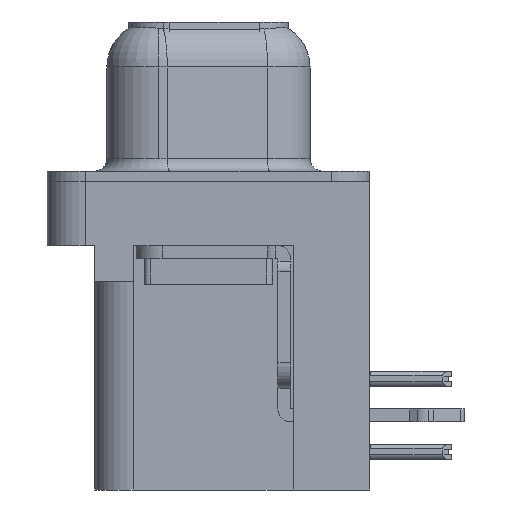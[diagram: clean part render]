
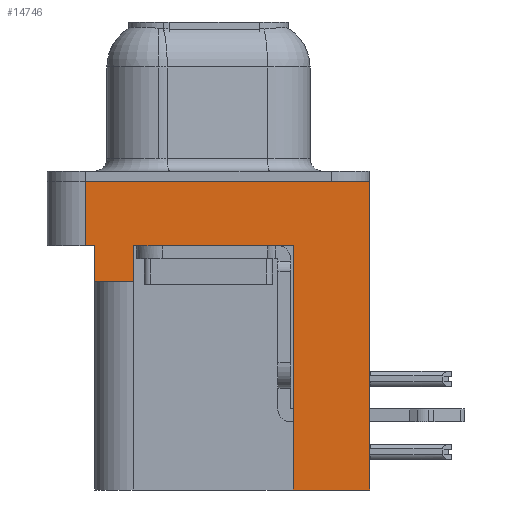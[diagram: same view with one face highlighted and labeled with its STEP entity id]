
A CAD part, left-side view. The second image highlights one B-rep face of the part: STEP entity #14746.
In plain terms, the highlighted planar face has unit normal (-1, 0, 0).
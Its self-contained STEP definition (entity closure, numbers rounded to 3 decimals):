
#140 = CARTESIAN_POINT ( 'NONE',  ( -2.935, -3.295, -2.5 ) ) ;
#238 = DIRECTION ( 'NONE',  ( 0., 0., 1. ) ) ;
#507 = LINE ( 'NONE', #5532, #8918 ) ;
#726 = CARTESIAN_POINT ( 'NONE',  ( -2.935, -6.275, -2.5 ) ) ;
#1962 = VERTEX_POINT ( 'NONE', #24941 ) ;
#2239 = VERTEX_POINT ( 'NONE', #6977 ) ;
#2416 = ORIENTED_EDGE ( 'NONE', *, *, #14369, .F. ) ;
#2509 = EDGE_CURVE ( 'NONE', #13848, #7947, #21451, .T. ) ;
#2587 = LINE ( 'NONE', #9626, #4948 ) ;
#2781 = VECTOR ( 'NONE', #238, 1000. ) ;
#2790 = LINE ( 'NONE', #20715, #17519 ) ;
#3121 = ORIENTED_EDGE ( 'NONE', *, *, #6282, .T. ) ;
#3251 = CARTESIAN_POINT ( 'NONE',  ( -2.935, -3.295, -12. ) ) ;
#3507 = DIRECTION ( 'NONE',  ( 0., 1., 0. ) ) ;
#3618 = VECTOR ( 'NONE', #19946, 1000. ) ;
#3640 = CARTESIAN_POINT ( 'NONE',  ( -2.935, 2.895, -2.5 ) ) ;
#3683 = DIRECTION ( 'NONE',  ( 0., 0., 1. ) ) ;
#3917 = EDGE_CURVE ( 'NONE', #13127, #20764, #21679, .T. ) ;
#4265 = DIRECTION ( 'NONE',  ( 0., 0., 1. ) ) ;
#4433 = PLANE ( 'NONE',  #15944 ) ;
#4751 = LINE ( 'NONE', #10506, #11701 ) ;
#4853 = CARTESIAN_POINT ( 'NONE',  ( -2.935, 4.425, -3.9 ) ) ;
#4948 = VECTOR ( 'NONE', #19466, 1000. ) ;
#5463 = CARTESIAN_POINT ( 'NONE',  ( -2.935, 4.775, -2.5 ) ) ;
#5532 = CARTESIAN_POINT ( 'NONE',  ( -2.935, -6.275, -2.5 ) ) ;
#6073 = EDGE_CURVE ( 'NONE', #7947, #1962, #8695, .T. ) ;
#6282 = EDGE_CURVE ( 'NONE', #13848, #2239, #4751, .T. ) ;
#6315 = ORIENTED_EDGE ( 'NONE', *, *, #17492, .T. ) ;
#6928 = EDGE_LOOP ( 'NONE', ( #19329, #10002, #3121, #24791, #21638, #9398, #6315, #24312, #2416, #16852 ) ) ;
#6977 = CARTESIAN_POINT ( 'NONE',  ( -2.935, 4.425, -2.5 ) ) ;
#7828 = CARTESIAN_POINT ( 'NONE',  ( -2.935, 4.775, -2.5 ) ) ;
#7875 = VECTOR ( 'NONE', #22246, 1000. ) ;
#7947 = VERTEX_POINT ( 'NONE', #19661 ) ;
#8245 = LINE ( 'NONE', #18409, #19979 ) ;
#8695 = LINE ( 'NONE', #10614, #3618 ) ;
#8802 = CARTESIAN_POINT ( 'NONE',  ( -2.935, 4.425, -3.9 ) ) ;
#8918 = VECTOR ( 'NONE', #3683, 1000. ) ;
#9371 = FACE_OUTER_BOUND ( 'NONE', #6928, .T. ) ;
#9398 = ORIENTED_EDGE ( 'NONE', *, *, #3917, .T. ) ;
#9626 = CARTESIAN_POINT ( 'NONE',  ( -2.935, -3.295, -12. ) ) ;
#9820 = DIRECTION ( 'NONE',  ( 0., 0., 1. ) ) ;
#10002 = ORIENTED_EDGE ( 'NONE', *, *, #2509, .F. ) ;
#10506 = CARTESIAN_POINT ( 'NONE',  ( -2.935, -6.275, -2.5 ) ) ;
#10614 = CARTESIAN_POINT ( 'NONE',  ( -2.935, -6.275, 0. ) ) ;
#11242 = VECTOR ( 'NONE', #9820, 1000. ) ;
#11701 = VECTOR ( 'NONE', #18063, 1000. ) ;
#12180 = CARTESIAN_POINT ( 'NONE',  ( -2.935, -6.275, -12. ) ) ;
#13011 = LINE ( 'NONE', #8802, #7875 ) ;
#13127 = VERTEX_POINT ( 'NONE', #13925 ) ;
#13670 = CARTESIAN_POINT ( 'NONE',  ( -2.935, 2.895, -3.9 ) ) ;
#13848 = VERTEX_POINT ( 'NONE', #7828 ) ;
#13925 = CARTESIAN_POINT ( 'NONE',  ( -2.935, 2.895, -3.9 ) ) ;
#14369 = EDGE_CURVE ( 'NONE', #18572, #18640, #2790, .T. ) ;
#14418 = VERTEX_POINT ( 'NONE', #140 ) ;
#14746 = ADVANCED_FACE ( 'NONE', ( #9371 ), #4433, .T. ) ;
#15848 = DIRECTION ( 'NONE',  ( -1., 0., 0. ) ) ;
#15944 = AXIS2_PLACEMENT_3D ( 'NONE', #726, #15848, #4265 ) ;
#16317 = EDGE_CURVE ( 'NONE', #18572, #1962, #507, .T. ) ;
#16359 = EDGE_CURVE ( 'NONE', #18640, #14418, #2587, .T. ) ;
#16845 = DIRECTION ( 'NONE',  ( 0., 1., 0. ) ) ;
#16852 = ORIENTED_EDGE ( 'NONE', *, *, #16317, .T. ) ;
#17492 = EDGE_CURVE ( 'NONE', #20764, #14418, #8245, .T. ) ;
#17519 = VECTOR ( 'NONE', #3507, 1000. ) ;
#18063 = DIRECTION ( 'NONE',  ( 0., -1., 0. ) ) ;
#18361 = VECTOR ( 'NONE', #16845, 1000. ) ;
#18409 = CARTESIAN_POINT ( 'NONE',  ( -2.935, -6.275, -2.5 ) ) ;
#18572 = VERTEX_POINT ( 'NONE', #12180 ) ;
#18578 = DIRECTION ( 'NONE',  ( 0., -1., 0. ) ) ;
#18640 = VERTEX_POINT ( 'NONE', #3251 ) ;
#19329 = ORIENTED_EDGE ( 'NONE', *, *, #6073, .F. ) ;
#19466 = DIRECTION ( 'NONE',  ( 0., 0., 1. ) ) ;
#19661 = CARTESIAN_POINT ( 'NONE',  ( -2.935, 4.775, 0. ) ) ;
#19946 = DIRECTION ( 'NONE',  ( 0., -1., 0. ) ) ;
#19979 = VECTOR ( 'NONE', #18578, 1000. ) ;
#20413 = CARTESIAN_POINT ( 'NONE',  ( -2.935, 4.425, -3.9 ) ) ;
#20552 = EDGE_CURVE ( 'NONE', #13127, #23803, #22884, .T. ) ;
#20715 = CARTESIAN_POINT ( 'NONE',  ( -2.935, -3.295, -12. ) ) ;
#20764 = VERTEX_POINT ( 'NONE', #3640 ) ;
#21451 = LINE ( 'NONE', #5463, #11242 ) ;
#21638 = ORIENTED_EDGE ( 'NONE', *, *, #20552, .F. ) ;
#21679 = LINE ( 'NONE', #13670, #2781 ) ;
#22246 = DIRECTION ( 'NONE',  ( 0., 0., 1. ) ) ;
#22884 = LINE ( 'NONE', #20413, #18361 ) ;
#23274 = EDGE_CURVE ( 'NONE', #23803, #2239, #13011, .T. ) ;
#23803 = VERTEX_POINT ( 'NONE', #4853 ) ;
#24312 = ORIENTED_EDGE ( 'NONE', *, *, #16359, .F. ) ;
#24791 = ORIENTED_EDGE ( 'NONE', *, *, #23274, .F. ) ;
#24941 = CARTESIAN_POINT ( 'NONE',  ( -2.935, -6.275, 0. ) ) ;
